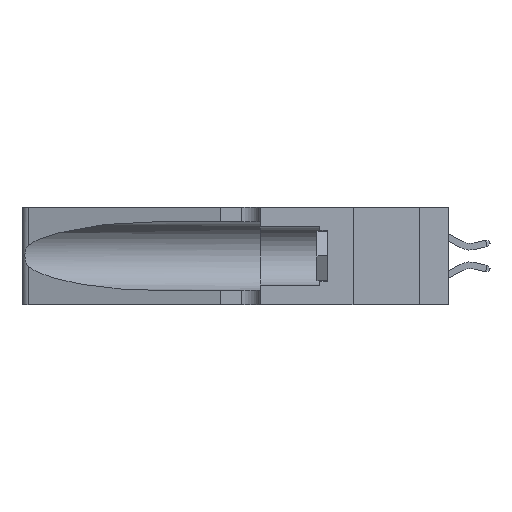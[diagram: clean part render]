
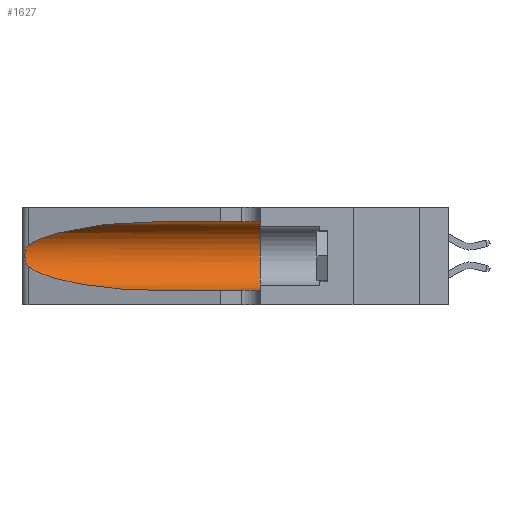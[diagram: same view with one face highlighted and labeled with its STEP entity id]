
A CAD part, left-side view. The second image highlights one B-rep face of the part: STEP entity #1627.
In plain terms, the highlighted cylindrical face has radius 3.308 mm (diameter 6.617 mm), a partial arc.
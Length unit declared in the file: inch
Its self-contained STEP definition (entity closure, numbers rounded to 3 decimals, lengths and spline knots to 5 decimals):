
#221 = CARTESIAN_POINT ( 'NONE',  ( 0.1305, 1.61858, 0.185 ) ) ;
#1248 = CARTESIAN_POINT ( 'NONE',  ( 0.25487, 1.22718, 0.14631 ) ) ;
#1627 = ADVANCED_FACE ( 'NONE', ( #15830 ), #13962, .F. ) ;
#3000 =( BOUNDED_CURVE ( )  B_SPLINE_CURVE ( 3, ( #11967, #35682, #15131, #35812 ),
 .UNSPECIFIED., .F., .F. ) 
 B_SPLINE_CURVE_WITH_KNOTS ( ( 4, 4 ),
 ( 3.44316, 4.71239 ),
 .UNSPECIFIED. ) 
 CURVE ( )  GEOMETRIC_REPRESENTATION_ITEM ( )  RATIONAL_B_SPLINE_CURVE ( ( 1., 0.87, 0.87, 1. ) ) 
 REPRESENTATION_ITEM ( '' )  );
#4046 = VERTEX_POINT ( 'NONE', #22100 ) ;
#4192 = CARTESIAN_POINT ( 'NONE',  ( 0.25639, 1.23184, 0.21858 ) ) ;
#4308 = CARTESIAN_POINT ( 'NONE',  ( 0.1305, 0.72297, 0.05475 ) ) ;
#4442 = CARTESIAN_POINT ( 'NONE',  ( 0.25487, 1.22718, 0.22369 ) ) ;
#4818 = EDGE_CURVE ( 'NONE', #28168, #4046, #33133, .T. ) ;
#5974 = B_SPLINE_CURVE_WITH_KNOTS ( 'NONE', 3,
 ( #16278, #33959, #4192, #25152, #7284, #28118, #10370, #31087, #13394, #34096, #16402, #37086, #19366, #1248 ),
 .UNSPECIFIED., .F., .F.,
 ( 4, 2, 2, 2, 2, 2, 4 ),
 ( 0., 0.00027, 0.00053, 0.00107, 0.0016, 0.00187, 0.00214 ),
 .UNSPECIFIED. ) ;
#6750 = VERTEX_POINT ( 'NONE', #4442 ) ;
#6873 = EDGE_CURVE ( 'NONE', #19884, #16879, #34945, .T. ) ;
#7284 = CARTESIAN_POINT ( 'NONE',  ( 0.25854, 1.2359, 0.20912 ) ) ;
#9507 = DIRECTION ( 'NONE',  ( 0., 0., -1. ) ) ;
#9769 = EDGE_LOOP ( 'NONE', ( #10922, #21561, #23905, #28088, #29463, #16146 ) ) ;
#10370 = CARTESIAN_POINT ( 'NONE',  ( 0.26075, 1.23896, 0.19203 ) ) ;
#10422 = VECTOR ( 'NONE', #37851, 39.37008 ) ;
#10746 = CARTESIAN_POINT ( 'NONE',  ( 0.18966, 0.96281, 0.31525 ) ) ;
#10922 = ORIENTED_EDGE ( 'NONE', *, *, #12817, .T. ) ;
#11967 = CARTESIAN_POINT ( 'NONE',  ( 0.25487, 1.22718, 0.14631 ) ) ;
#12817 = EDGE_CURVE ( 'NONE', #28168, #6750, #22265, .T. ) ;
#13394 = CARTESIAN_POINT ( 'NONE',  ( 0.26017, 1.23833, 0.17102 ) ) ;
#13962 = CYLINDRICAL_SURFACE ( 'NONE', #28192, 0.13025 ) ;
#13964 = CARTESIAN_POINT ( 'NONE',  ( 0.1305, 0.72297, 0.31525 ) ) ;
#14167 = DIRECTION ( 'NONE',  ( 0., -1., 0. ) ) ;
#14978 = CARTESIAN_POINT ( 'NONE',  ( 0.1305, 0.35, 0.185 ) ) ;
#15131 = CARTESIAN_POINT ( 'NONE',  ( 0.18966, 0.96281, 0.05475 ) ) ;
#15830 = FACE_OUTER_BOUND ( 'NONE', #9769, .T. ) ;
#16146 = ORIENTED_EDGE ( 'NONE', *, *, #4818, .F. ) ;
#16278 = CARTESIAN_POINT ( 'NONE',  ( 0.25487, 1.22718, 0.22369 ) ) ;
#16402 = CARTESIAN_POINT ( 'NONE',  ( 0.25789, 1.23486, 0.15765 ) ) ;
#16755 = CARTESIAN_POINT ( 'NONE',  ( 0.2373, 1.15595, 0.28018 ) ) ;
#16879 = VERTEX_POINT ( 'NONE', #32454 ) ;
#17943 = DIRECTION ( 'NONE',  ( 0., 0., 1. ) ) ;
#18500 = CIRCLE ( 'NONE', #29375, 0.13025 ) ;
#19366 = CARTESIAN_POINT ( 'NONE',  ( 0.25555, 1.22993, 0.14849 ) ) ;
#19884 = VERTEX_POINT ( 'NONE', #4308 ) ;
#20120 = CARTESIAN_POINT ( 'NONE',  ( 0.1305, 1.61858, 0.31525 ) ) ;
#21561 = ORIENTED_EDGE ( 'NONE', *, *, #33585, .T. ) ;
#22100 = CARTESIAN_POINT ( 'NONE',  ( 0.1305, 0.35, 0.31525 ) ) ;
#22265 =( BOUNDED_CURVE ( )  B_SPLINE_CURVE ( 3, ( #31447, #10746, #16755, #37434 ),
 .UNSPECIFIED., .F., .F. ) 
 B_SPLINE_CURVE_WITH_KNOTS ( ( 4, 4 ),
 ( 1.5708, 2.84003 ),
 .UNSPECIFIED. ) 
 CURVE ( )  GEOMETRIC_REPRESENTATION_ITEM ( )  RATIONAL_B_SPLINE_CURVE ( ( 1., 0.87, 0.87, 1. ) ) 
 REPRESENTATION_ITEM ( '' )  );
#23905 = ORIENTED_EDGE ( 'NONE', *, *, #26429, .T. ) ;
#25152 = CARTESIAN_POINT ( 'NONE',  ( 0.25787, 1.23484, 0.2124 ) ) ;
#25346 = CARTESIAN_POINT ( 'NONE',  ( 0.25487, 1.22718, 0.14631 ) ) ;
#26429 = EDGE_CURVE ( 'NONE', #30200, #19884, #3000, .T. ) ;
#27266 = DIRECTION ( 'NONE',  ( 0., -1., 0. ) ) ;
#28088 = ORIENTED_EDGE ( 'NONE', *, *, #6873, .T. ) ;
#28118 = CARTESIAN_POINT ( 'NONE',  ( 0.26018, 1.23835, 0.19895 ) ) ;
#28168 = VERTEX_POINT ( 'NONE', #13964 ) ;
#28192 = AXIS2_PLACEMENT_3D ( 'NONE', #221, #27266, #9507 ) ;
#29375 = AXIS2_PLACEMENT_3D ( 'NONE', #14978, #35663, #17943 ) ;
#29463 = ORIENTED_EDGE ( 'NONE', *, *, #31349, .F. ) ;
#30200 = VERTEX_POINT ( 'NONE', #25346 ) ;
#31087 = CARTESIAN_POINT ( 'NONE',  ( 0.26075, 1.23896, 0.178 ) ) ;
#31349 = EDGE_CURVE ( 'NONE', #4046, #16879, #18500, .T. ) ;
#31447 = CARTESIAN_POINT ( 'NONE',  ( 0.1305, 0.72297, 0.31525 ) ) ;
#31737 = CARTESIAN_POINT ( 'NONE',  ( 0.1305, 1.61858, 0.05475 ) ) ;
#32454 = CARTESIAN_POINT ( 'NONE',  ( 0.1305, 0.35, 0.05475 ) ) ;
#33133 = LINE ( 'NONE', #20120, #10422 ) ;
#33585 = EDGE_CURVE ( 'NONE', #6750, #30200, #5974, .T. ) ;
#33959 = CARTESIAN_POINT ( 'NONE',  ( 0.25555, 1.22994, 0.2215 ) ) ;
#34008 = VECTOR ( 'NONE', #14167, 39.37008 ) ;
#34096 = CARTESIAN_POINT ( 'NONE',  ( 0.25856, 1.23593, 0.16098 ) ) ;
#34945 = LINE ( 'NONE', #31737, #34008 ) ;
#35663 = DIRECTION ( 'NONE',  ( 0., 1., 0. ) ) ;
#35682 = CARTESIAN_POINT ( 'NONE',  ( 0.2373, 1.15595, 0.08982 ) ) ;
#35812 = CARTESIAN_POINT ( 'NONE',  ( 0.1305, 0.72297, 0.05475 ) ) ;
#37086 = CARTESIAN_POINT ( 'NONE',  ( 0.25639, 1.23186, 0.15144 ) ) ;
#37434 = CARTESIAN_POINT ( 'NONE',  ( 0.25487, 1.22718, 0.22369 ) ) ;
#37851 = DIRECTION ( 'NONE',  ( 0., -1., 0. ) ) ;
